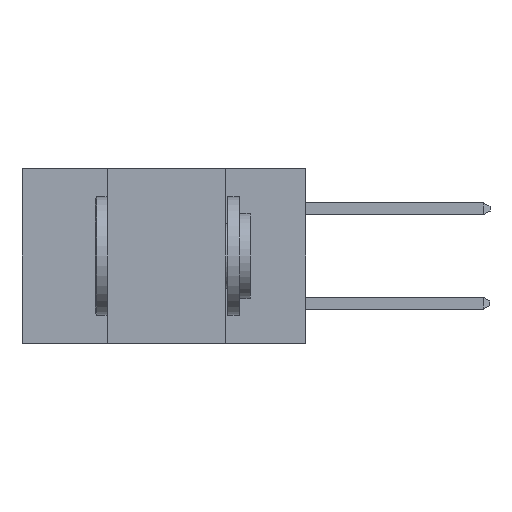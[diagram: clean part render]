
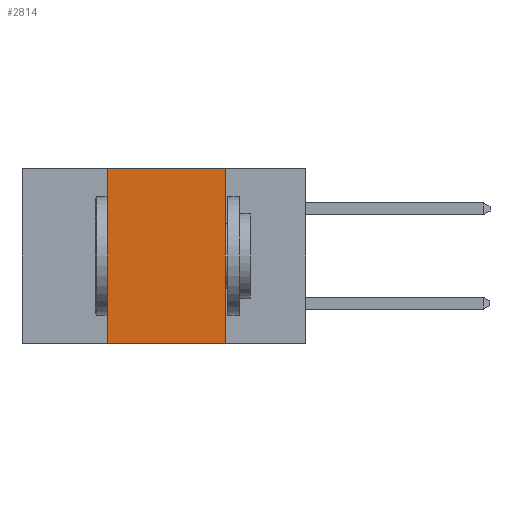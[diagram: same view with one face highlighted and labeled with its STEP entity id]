
A CAD part, left-side view. The second image highlights one B-rep face of the part: STEP entity #2814.
In plain terms, the highlighted planar face has unit normal (-1, 0, 0).
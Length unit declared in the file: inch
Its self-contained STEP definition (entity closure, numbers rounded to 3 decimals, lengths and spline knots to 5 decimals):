
#761 = VERTEX_POINT ( 'NONE', #15675 ) ;
#1325 = LINE ( 'NONE', #7608, #11251 ) ;
#1507 = VECTOR ( 'NONE', #6080, 39.37008 ) ;
#2814 = ADVANCED_FACE ( 'NONE', ( #15785 ), #6027, .F. ) ;
#2992 = VERTEX_POINT ( 'NONE', #5184 ) ;
#3005 = EDGE_CURVE ( 'NONE', #2992, #8129, #13159, .T. ) ;
#3139 = CARTESIAN_POINT ( 'NONE',  ( 0., 0.17, 0. ) ) ;
#3157 = CARTESIAN_POINT ( 'NONE',  ( 0., 0.17, -0.37 ) ) ;
#3604 = EDGE_LOOP ( 'NONE', ( #4034, #13458, #6589, #11368 ) ) ;
#4027 = EDGE_CURVE ( 'NONE', #4312, #8129, #1325, .T. ) ;
#4034 = ORIENTED_EDGE ( 'NONE', *, *, #4027, .F. ) ;
#4312 = VERTEX_POINT ( 'NONE', #3139 ) ;
#4705 = LINE ( 'NONE', #12297, #7212 ) ;
#5184 = CARTESIAN_POINT ( 'NONE',  ( 0., 0.42, -0.37 ) ) ;
#6027 = PLANE ( 'NONE',  #13139 ) ;
#6080 = DIRECTION ( 'NONE',  ( 0., 0., 1. ) ) ;
#6589 = ORIENTED_EDGE ( 'NONE', *, *, #15286, .F. ) ;
#7212 = VECTOR ( 'NONE', #13511, 39.37008 ) ;
#7608 = CARTESIAN_POINT ( 'NONE',  ( 0., 0.17, 0. ) ) ;
#8064 = DIRECTION ( 'NONE',  ( 0., 0., -1. ) ) ;
#8129 = VERTEX_POINT ( 'NONE', #3157 ) ;
#8137 = LINE ( 'NONE', #13390, #1507 ) ;
#9552 = DIRECTION ( 'NONE',  ( 0., 0., -1. ) ) ;
#10015 = CARTESIAN_POINT ( 'NONE',  ( 0., 0.6, -0.37 ) ) ;
#10253 = DIRECTION ( 'NONE',  ( 0., -1., 0. ) ) ;
#10282 = VECTOR ( 'NONE', #10253, 39.37008 ) ;
#11251 = VECTOR ( 'NONE', #8064, 39.37008 ) ;
#11368 = ORIENTED_EDGE ( 'NONE', *, *, #3005, .T. ) ;
#12297 = CARTESIAN_POINT ( 'NONE',  ( 0., 0.6, 0. ) ) ;
#13139 = AXIS2_PLACEMENT_3D ( 'NONE', #15603, #14279, #9552 ) ;
#13159 = LINE ( 'NONE', #10015, #10282 ) ;
#13390 = CARTESIAN_POINT ( 'NONE',  ( 0., 0.42, 0. ) ) ;
#13458 = ORIENTED_EDGE ( 'NONE', *, *, #14665, .F. ) ;
#13511 = DIRECTION ( 'NONE',  ( 0., -1., 0. ) ) ;
#14279 = DIRECTION ( 'NONE',  ( 1., 0., 0. ) ) ;
#14665 = EDGE_CURVE ( 'NONE', #761, #4312, #4705, .T. ) ;
#15286 = EDGE_CURVE ( 'NONE', #2992, #761, #8137, .T. ) ;
#15603 = CARTESIAN_POINT ( 'NONE',  ( 0., 0.6, 0. ) ) ;
#15675 = CARTESIAN_POINT ( 'NONE',  ( 0., 0.42, 0. ) ) ;
#15785 = FACE_OUTER_BOUND ( 'NONE', #3604, .T. ) ;
